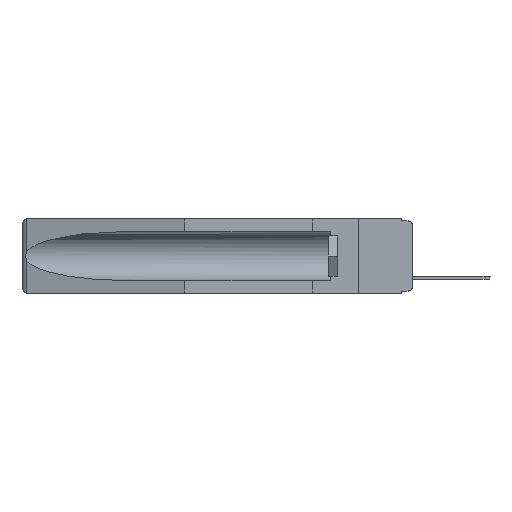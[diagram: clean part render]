
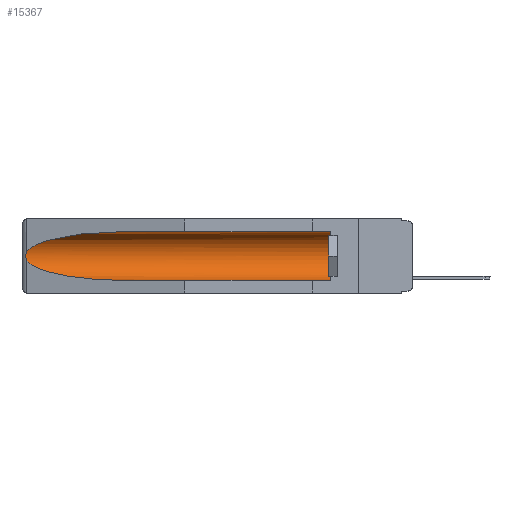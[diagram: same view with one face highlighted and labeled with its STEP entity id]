
A CAD part, left-side view. The second image highlights one B-rep face of the part: STEP entity #15367.
In plain terms, the highlighted cylindrical face has radius 2.857 mm (diameter 5.715 mm), a partial arc.
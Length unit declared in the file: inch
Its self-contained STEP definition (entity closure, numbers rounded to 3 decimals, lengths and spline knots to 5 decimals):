
#520 = CARTESIAN_POINT ( 'NONE',  ( 0.2675, 1.53308, -0.17534 ) ) ;
#716 = CARTESIAN_POINT ( 'NONE',  ( 0.26537, 1.52718, -0.14972 ) ) ;
#1381 = CARTESIAN_POINT ( 'NONE',  ( 0.155, 1.07973, -0.059 ) ) ;
#1588 = VERTEX_POINT ( 'NONE', #3157 ) ;
#1625 = ORIENTED_EDGE ( 'NONE', *, *, #13731, .T. ) ;
#2047 = CYLINDRICAL_SURFACE ( 'NONE', #5182, 0.1125 ) ;
#2135 = CARTESIAN_POINT ( 'NONE',  ( 0.155, 0.126, -0.059 ) ) ;
#2203 = EDGE_CURVE ( 'NONE', #19579, #13797, #5204, .T. ) ;
#2655 = CARTESIAN_POINT ( 'NONE',  ( 0.21114, 1.30732, -0.284 ) ) ;
#2816 = B_SPLINE_CURVE_WITH_KNOTS ( 'NONE', 3,
 ( #716, #7147, #18517, #10418, #16750, #520, #5386, #18229, #10519, #7044 ),
 .UNSPECIFIED., .F., .F.,
 ( 4, 2, 2, 2, 4 ),
 ( 0., 0.00029, 0.00058, 0.00087, 0.00117 ),
 .UNSPECIFIED. ) ;
#2919 = EDGE_CURVE ( 'NONE', #7135, #19579, #2816, .T. ) ;
#3157 = CARTESIAN_POINT ( 'NONE',  ( 0.155, 0.126, -0.284 ) ) ;
#3630 = FACE_OUTER_BOUND ( 'NONE', #16529, .T. ) ;
#4541 = CARTESIAN_POINT ( 'NONE',  ( 0.21114, 1.30732, -0.059 ) ) ;
#5001 = VERTEX_POINT ( 'NONE', #2135 ) ;
#5059 = CARTESIAN_POINT ( 'NONE',  ( 0.155, -0.30754, -0.059 ) ) ;
#5099 = ORIENTED_EDGE ( 'NONE', *, *, #8499, .T. ) ;
#5182 = AXIS2_PLACEMENT_3D ( 'NONE', #19849, #5339, #11737 ) ;
#5204 =( BOUNDED_CURVE ( )  B_SPLINE_CURVE ( 3, ( #10781, #15940, #2655, #7604 ),
 .UNSPECIFIED., .F., .F. ) 
 B_SPLINE_CURVE_WITH_KNOTS ( ( 4, 4 ),
 ( 0.1948, 1.5708 ),
 .UNSPECIFIED. ) 
 CURVE ( )  GEOMETRIC_REPRESENTATION_ITEM ( )  RATIONAL_B_SPLINE_CURVE ( ( 1., 0.848, 0.848, 1. ) ) 
 REPRESENTATION_ITEM ( '' )  );
#5283 = VERTEX_POINT ( 'NONE', #1381 ) ;
#5339 = DIRECTION ( 'NONE',  ( 0., 1., 0. ) ) ;
#5386 = CARTESIAN_POINT ( 'NONE',  ( 0.2673, 1.53269, -0.17917 ) ) ;
#5642 = CARTESIAN_POINT ( 'NONE',  ( 0.155, -0.30754, -0.284 ) ) ;
#5769 = AXIS2_PLACEMENT_3D ( 'NONE', #6177, #10923, #20168 ) ;
#6177 = CARTESIAN_POINT ( 'NONE',  ( 0.155, 0.126, -0.1715 ) ) ;
#6258 = ORIENTED_EDGE ( 'NONE', *, *, #11250, .T. ) ;
#6323 = CARTESIAN_POINT ( 'NONE',  ( 0.26537, 1.52718, -0.14972 ) ) ;
#7044 = CARTESIAN_POINT ( 'NONE',  ( 0.26537, 1.52718, -0.19328 ) ) ;
#7135 = VERTEX_POINT ( 'NONE', #12741 ) ;
#7147 = CARTESIAN_POINT ( 'NONE',  ( 0.26597, 1.52961, -0.15275 ) ) ;
#7604 = CARTESIAN_POINT ( 'NONE',  ( 0.155, 1.07973, -0.284 ) ) ;
#7783 = CIRCLE ( 'NONE', #5769, 0.1125 ) ;
#8499 = EDGE_CURVE ( 'NONE', #5001, #5283, #14424, .T. ) ;
#8888 = VECTOR ( 'NONE', #15223, 39.37008 ) ;
#10418 = CARTESIAN_POINT ( 'NONE',  ( 0.2673, 1.5327, -0.16383 ) ) ;
#10519 = CARTESIAN_POINT ( 'NONE',  ( 0.26597, 1.5296, -0.19026 ) ) ;
#10781 = CARTESIAN_POINT ( 'NONE',  ( 0.26537, 1.52718, -0.19328 ) ) ;
#10923 = DIRECTION ( 'NONE',  ( 0., -1., 0. ) ) ;
#11250 = EDGE_CURVE ( 'NONE', #5283, #7135, #13300, .T. ) ;
#11737 = DIRECTION ( 'NONE',  ( 0., 0., 1. ) ) ;
#12741 = CARTESIAN_POINT ( 'NONE',  ( 0.26537, 1.52718, -0.14972 ) ) ;
#13126 = ORIENTED_EDGE ( 'NONE', *, *, #2919, .T. ) ;
#13300 =( BOUNDED_CURVE ( )  B_SPLINE_CURVE ( 3, ( #17070, #4541, #20737, #6323 ),
 .UNSPECIFIED., .F., .F. ) 
 B_SPLINE_CURVE_WITH_KNOTS ( ( 4, 4 ),
 ( 4.71239, 6.08839 ),
 .UNSPECIFIED. ) 
 CURVE ( )  GEOMETRIC_REPRESENTATION_ITEM ( )  RATIONAL_B_SPLINE_CURVE ( ( 1., 0.848, 0.848, 1. ) ) 
 REPRESENTATION_ITEM ( '' )  );
#13731 = EDGE_CURVE ( 'NONE', #1588, #5001, #7783, .T. ) ;
#13797 = VERTEX_POINT ( 'NONE', #20274 ) ;
#13844 = ORIENTED_EDGE ( 'NONE', *, *, #2203, .T. ) ;
#14424 = LINE ( 'NONE', #5059, #15020 ) ;
#15020 = VECTOR ( 'NONE', #19267, 39.37008 ) ;
#15223 = DIRECTION ( 'NONE',  ( 0., 1., 0. ) ) ;
#15367 = ADVANCED_FACE ( 'NONE', ( #3630 ), #2047, .F. ) ;
#15940 = CARTESIAN_POINT ( 'NONE',  ( 0.25451, 1.48313, -0.24835 ) ) ;
#16529 = EDGE_LOOP ( 'NONE', ( #6258, #13126, #13844, #19777, #1625, #5099 ) ) ;
#16572 = EDGE_CURVE ( 'NONE', #1588, #13797, #20148, .T. ) ;
#16750 = CARTESIAN_POINT ( 'NONE',  ( 0.2675, 1.53308, -0.16763 ) ) ;
#17070 = CARTESIAN_POINT ( 'NONE',  ( 0.155, 1.07973, -0.059 ) ) ;
#18229 = CARTESIAN_POINT ( 'NONE',  ( 0.26655, 1.53094, -0.18657 ) ) ;
#18517 = CARTESIAN_POINT ( 'NONE',  ( 0.26654, 1.53092, -0.15636 ) ) ;
#18657 = CARTESIAN_POINT ( 'NONE',  ( 0.26537, 1.52718, -0.19328 ) ) ;
#19267 = DIRECTION ( 'NONE',  ( 0., 1., 0. ) ) ;
#19579 = VERTEX_POINT ( 'NONE', #18657 ) ;
#19777 = ORIENTED_EDGE ( 'NONE', *, *, #16572, .F. ) ;
#19849 = CARTESIAN_POINT ( 'NONE',  ( 0.155, -0.30754, -0.1715 ) ) ;
#20148 = LINE ( 'NONE', #5642, #8888 ) ;
#20168 = DIRECTION ( 'NONE',  ( 0., 0., 1. ) ) ;
#20274 = CARTESIAN_POINT ( 'NONE',  ( 0.155, 1.07973, -0.284 ) ) ;
#20737 = CARTESIAN_POINT ( 'NONE',  ( 0.25451, 1.48313, -0.09465 ) ) ;
